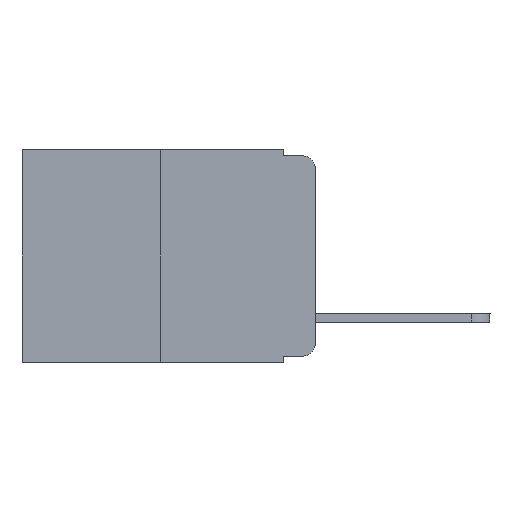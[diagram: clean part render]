
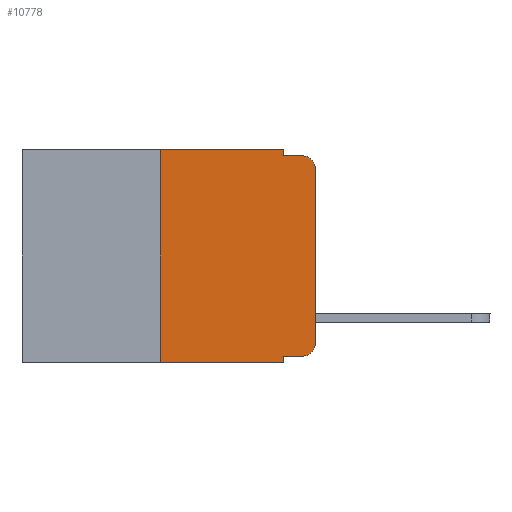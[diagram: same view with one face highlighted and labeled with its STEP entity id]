
A CAD part, left-side view. The second image highlights one B-rep face of the part: STEP entity #10778.
In plain terms, the highlighted planar face has unit normal (-1, 0, 0).
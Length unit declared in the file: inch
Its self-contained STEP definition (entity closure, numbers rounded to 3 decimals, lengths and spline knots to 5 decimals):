
#46 = CIRCLE ( 'NONE', #8125, 0.02 ) ;
#128 = CIRCLE ( 'NONE', #9937, 0.02 ) ;
#168 = DIRECTION ( 'NONE',  ( 0., -1., 0. ) ) ;
#223 = DIRECTION ( 'NONE',  ( 1., 0., 0. ) ) ;
#266 = CARTESIAN_POINT ( 'NONE',  ( 0., 0.051, -0.333 ) ) ;
#738 = DIRECTION ( 'NONE',  ( 0., -1., 0. ) ) ;
#1397 = ORIENTED_EDGE ( 'NONE', *, *, #3876, .F. ) ;
#1439 = EDGE_CURVE ( 'NONE', #2619, #9726, #46, .T. ) ;
#1501 = DIRECTION ( 'NONE',  ( 0., 0., 1. ) ) ;
#1540 = CARTESIAN_POINT ( 'NONE',  ( 0., 0., 0. ) ) ;
#1641 = CARTESIAN_POINT ( 'NONE',  ( 0., 0.473, 0. ) ) ;
#1731 = VECTOR ( 'NONE', #2401, 39.37008 ) ;
#2281 = EDGE_CURVE ( 'NONE', #7512, #5757, #10322, .T. ) ;
#2337 = EDGE_CURVE ( 'NONE', #5757, #10937, #128, .T. ) ;
#2401 = DIRECTION ( 'NONE',  ( 0., -1., 0. ) ) ;
#2617 = CARTESIAN_POINT ( 'NONE',  ( 0., 0.051, -0.343 ) ) ;
#2619 = VERTEX_POINT ( 'NONE', #4455 ) ;
#2657 = ORIENTED_EDGE ( 'NONE', *, *, #4380, .T. ) ;
#3052 = ORIENTED_EDGE ( 'NONE', *, *, #11463, .F. ) ;
#3313 = LINE ( 'NONE', #11456, #11854 ) ;
#3448 = LINE ( 'NONE', #4845, #4466 ) ;
#3694 = EDGE_LOOP ( 'NONE', ( #2657, #3942, #5818, #4566, #1397, #3052, #11048, #6078, #9253, #6505 ) ) ;
#3876 = EDGE_CURVE ( 'NONE', #7975, #9982, #8236, .T. ) ;
#3942 = ORIENTED_EDGE ( 'NONE', *, *, #1439, .T. ) ;
#3949 = DIRECTION ( 'NONE',  ( 0., 0., -1. ) ) ;
#3977 = CARTESIAN_POINT ( 'NONE',  ( 0., 0.02, -0.313 ) ) ;
#4068 = LINE ( 'NONE', #1540, #9979 ) ;
#4082 = VECTOR ( 'NONE', #6820, 39.37008 ) ;
#4314 = EDGE_CURVE ( 'NONE', #9982, #8795, #7502, .T. ) ;
#4380 = EDGE_CURVE ( 'NONE', #10937, #2619, #4068, .T. ) ;
#4429 = EDGE_CURVE ( 'NONE', #8795, #9726, #9829, .T. ) ;
#4455 = CARTESIAN_POINT ( 'NONE',  ( 0., 0., -0.03 ) ) ;
#4466 = VECTOR ( 'NONE', #9820, 39.37008 ) ;
#4485 = AXIS2_PLACEMENT_3D ( 'NONE', #7618, #223, #3949 ) ;
#4566 = ORIENTED_EDGE ( 'NONE', *, *, #4314, .F. ) ;
#4613 = DIRECTION ( 'NONE',  ( 0., 0., -1. ) ) ;
#4845 = CARTESIAN_POINT ( 'NONE',  ( 0., 0.25, 0. ) ) ;
#5124 = CARTESIAN_POINT ( 'NONE',  ( 0., 0.051, -0.01 ) ) ;
#5265 = CARTESIAN_POINT ( 'NONE',  ( 0., 0., -0.313 ) ) ;
#5437 = EDGE_CURVE ( 'NONE', #8932, #11021, #3313, .T. ) ;
#5503 = CARTESIAN_POINT ( 'NONE',  ( 0., 0.02, -0.03 ) ) ;
#5553 = DIRECTION ( 'NONE',  ( 0., -1., 0. ) ) ;
#5663 = CARTESIAN_POINT ( 'NONE',  ( 0., 0.051, -0.01 ) ) ;
#5757 = VERTEX_POINT ( 'NONE', #7310 ) ;
#5818 = ORIENTED_EDGE ( 'NONE', *, *, #4429, .F. ) ;
#6078 = ORIENTED_EDGE ( 'NONE', *, *, #6234, .F. ) ;
#6234 = EDGE_CURVE ( 'NONE', #7512, #11021, #8583, .T. ) ;
#6263 = DIRECTION ( 'NONE',  ( 0., 0., -1. ) ) ;
#6304 = CARTESIAN_POINT ( 'NONE',  ( 0., 0.051, 0. ) ) ;
#6505 = ORIENTED_EDGE ( 'NONE', *, *, #2337, .T. ) ;
#6820 = DIRECTION ( 'NONE',  ( 0., 0., -1. ) ) ;
#7310 = CARTESIAN_POINT ( 'NONE',  ( 0., 0.02, -0.333 ) ) ;
#7502 = LINE ( 'NONE', #8829, #4082 ) ;
#7512 = VERTEX_POINT ( 'NONE', #266 ) ;
#7588 = CARTESIAN_POINT ( 'NONE',  ( 0., 0.25, -0.343 ) ) ;
#7618 = CARTESIAN_POINT ( 'NONE',  ( 0., 0.473, 0. ) ) ;
#7953 = VECTOR ( 'NONE', #5553, 39.37008 ) ;
#7975 = VERTEX_POINT ( 'NONE', #8793 ) ;
#8125 = AXIS2_PLACEMENT_3D ( 'NONE', #5503, #10224, #4613 ) ;
#8236 = LINE ( 'NONE', #1641, #9695 ) ;
#8583 = LINE ( 'NONE', #6304, #10668 ) ;
#8631 = PLANE ( 'NONE',  #4485 ) ;
#8793 = CARTESIAN_POINT ( 'NONE',  ( 0., 0.25, 0. ) ) ;
#8795 = VERTEX_POINT ( 'NONE', #5663 ) ;
#8829 = CARTESIAN_POINT ( 'NONE',  ( 0., 0.051, 0. ) ) ;
#8932 = VERTEX_POINT ( 'NONE', #7588 ) ;
#9253 = ORIENTED_EDGE ( 'NONE', *, *, #2281, .T. ) ;
#9356 = FACE_OUTER_BOUND ( 'NONE', #3694, .T. ) ;
#9401 = DIRECTION ( 'NONE',  ( -1., 0., 0. ) ) ;
#9695 = VECTOR ( 'NONE', #738, 39.37008 ) ;
#9726 = VERTEX_POINT ( 'NONE', #10087 ) ;
#9820 = DIRECTION ( 'NONE',  ( 0., 0., 1. ) ) ;
#9829 = LINE ( 'NONE', #5124, #1731 ) ;
#9937 = AXIS2_PLACEMENT_3D ( 'NONE', #3977, #9401, #10653 ) ;
#9979 = VECTOR ( 'NONE', #1501, 39.37008 ) ;
#9982 = VERTEX_POINT ( 'NONE', #10314 ) ;
#10087 = CARTESIAN_POINT ( 'NONE',  ( 0., 0.02, -0.01 ) ) ;
#10224 = DIRECTION ( 'NONE',  ( -1., 0., 0. ) ) ;
#10276 = CARTESIAN_POINT ( 'NONE',  ( 0., 0.051, -0.333 ) ) ;
#10314 = CARTESIAN_POINT ( 'NONE',  ( 0., 0.051, 0. ) ) ;
#10322 = LINE ( 'NONE', #10276, #7953 ) ;
#10653 = DIRECTION ( 'NONE',  ( 0., 0., -1. ) ) ;
#10668 = VECTOR ( 'NONE', #6263, 39.37008 ) ;
#10778 = ADVANCED_FACE ( 'NONE', ( #9356 ), #8631, .F. ) ;
#10937 = VERTEX_POINT ( 'NONE', #5265 ) ;
#11021 = VERTEX_POINT ( 'NONE', #2617 ) ;
#11048 = ORIENTED_EDGE ( 'NONE', *, *, #5437, .T. ) ;
#11456 = CARTESIAN_POINT ( 'NONE',  ( 0., 0.473, -0.343 ) ) ;
#11463 = EDGE_CURVE ( 'NONE', #8932, #7975, #3448, .T. ) ;
#11854 = VECTOR ( 'NONE', #168, 39.37008 ) ;
